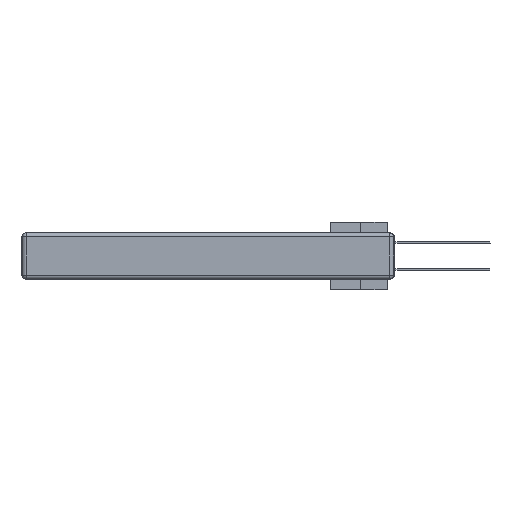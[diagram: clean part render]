
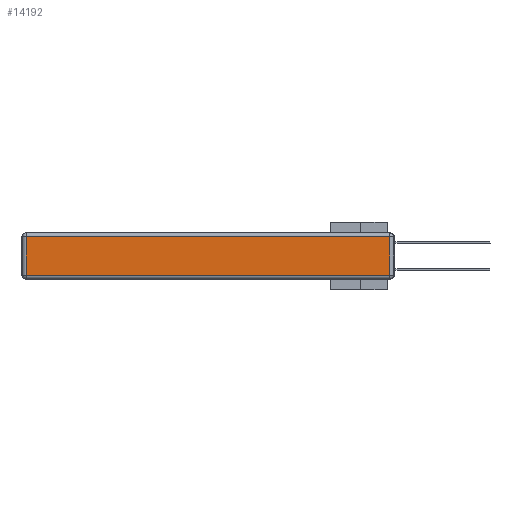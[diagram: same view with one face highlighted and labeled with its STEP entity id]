
A CAD part, left-side view. The second image highlights one B-rep face of the part: STEP entity #14192.
In plain terms, the highlighted planar face has unit normal (-1, 0, 0).
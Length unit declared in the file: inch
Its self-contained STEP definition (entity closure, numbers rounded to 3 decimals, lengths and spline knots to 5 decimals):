
#3377 = EDGE_CURVE ( 'NONE', #18980, #15723, #3689, .T. ) ;
#3520 = EDGE_LOOP ( 'NONE', ( #10162, #7229, #4139, #16375 ) ) ;
#3689 = LINE ( 'NONE', #9023, #6246 ) ;
#4139 = ORIENTED_EDGE ( 'NONE', *, *, #17723, .T. ) ;
#4801 = LINE ( 'NONE', #24714, #10273 ) ;
#5482 = DIRECTION ( 'NONE',  ( -1., 0., 0. ) ) ;
#5876 = CARTESIAN_POINT ( 'NONE',  ( 0., 2.72, -0.03 ) ) ;
#6246 = VECTOR ( 'NONE', #25443, 39.37008 ) ;
#7229 = ORIENTED_EDGE ( 'NONE', *, *, #3377, .T. ) ;
#7698 = DIRECTION ( 'NONE',  ( 0., 0., 1. ) ) ;
#8131 = VERTEX_POINT ( 'NONE', #5876 ) ;
#8369 = DIRECTION ( 'NONE',  ( 0., 0., -1. ) ) ;
#8428 = VERTEX_POINT ( 'NONE', #13084 ) ;
#9023 = CARTESIAN_POINT ( 'NONE',  ( 0., 0.03, -0.343 ) ) ;
#9074 = VECTOR ( 'NONE', #8369, 39.37008 ) ;
#10017 = CARTESIAN_POINT ( 'NONE',  ( 0., 0.03, -0.03 ) ) ;
#10162 = ORIENTED_EDGE ( 'NONE', *, *, #11447, .T. ) ;
#10273 = VECTOR ( 'NONE', #15365, 39.37008 ) ;
#10524 = CARTESIAN_POINT ( 'NONE',  ( 0., 0.03, -0.313 ) ) ;
#10665 = LINE ( 'NONE', #17806, #16469 ) ;
#11259 = LINE ( 'NONE', #20002, #9074 ) ;
#11447 = EDGE_CURVE ( 'NONE', #8428, #18980, #10665, .T. ) ;
#12359 = PLANE ( 'NONE',  #21619 ) ;
#13084 = CARTESIAN_POINT ( 'NONE',  ( 0., 2.72, -0.313 ) ) ;
#14192 = ADVANCED_FACE ( 'NONE', ( #18119 ), #12359, .T. ) ;
#15130 = DIRECTION ( 'NONE',  ( 0., -1., 0. ) ) ;
#15365 = DIRECTION ( 'NONE',  ( 0., 1., 0. ) ) ;
#15723 = VERTEX_POINT ( 'NONE', #10017 ) ;
#16375 = ORIENTED_EDGE ( 'NONE', *, *, #19040, .T. ) ;
#16469 = VECTOR ( 'NONE', #15130, 39.37008 ) ;
#17723 = EDGE_CURVE ( 'NONE', #15723, #8131, #4801, .T. ) ;
#17806 = CARTESIAN_POINT ( 'NONE',  ( 0., 0., -0.313 ) ) ;
#18119 = FACE_OUTER_BOUND ( 'NONE', #3520, .T. ) ;
#18980 = VERTEX_POINT ( 'NONE', #10524 ) ;
#19040 = EDGE_CURVE ( 'NONE', #8131, #8428, #11259, .T. ) ;
#20002 = CARTESIAN_POINT ( 'NONE',  ( 0., 2.72, -0.343 ) ) ;
#21619 = AXIS2_PLACEMENT_3D ( 'NONE', #26460, #5482, #7698 ) ;
#24714 = CARTESIAN_POINT ( 'NONE',  ( 0., 2.75, -0.03 ) ) ;
#25443 = DIRECTION ( 'NONE',  ( 0., 0., 1. ) ) ;
#26460 = CARTESIAN_POINT ( 'NONE',  ( 0., 0., -0.343 ) ) ;
